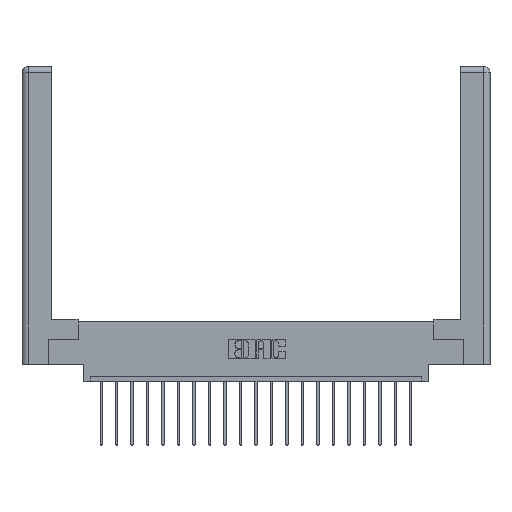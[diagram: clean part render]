
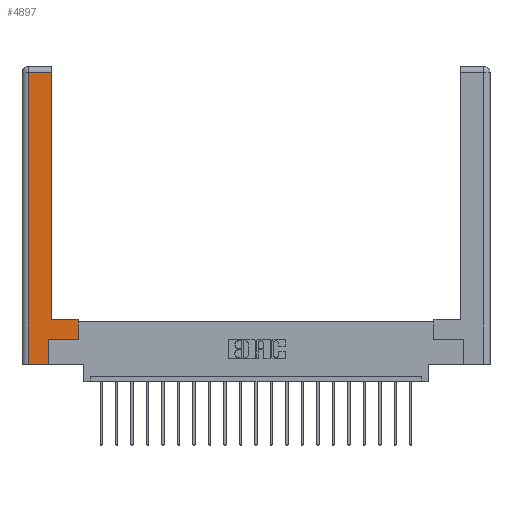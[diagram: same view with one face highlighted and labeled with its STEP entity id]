
A CAD part, top view. The second image highlights one B-rep face of the part: STEP entity #4897.
In plain terms, the highlighted planar face has unit normal (0, 0, 1).
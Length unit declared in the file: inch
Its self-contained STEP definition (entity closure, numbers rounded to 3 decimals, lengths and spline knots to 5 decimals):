
#216 = DIRECTION ( 'NONE',  ( 0., 1., 0. ) ) ;
#342 = DIRECTION ( 'NONE',  ( -1., 0., 0. ) ) ;
#1109 = LINE ( 'NONE', #13884, #18194 ) ;
#1409 = PLANE ( 'NONE',  #10050 ) ;
#1915 = EDGE_CURVE ( 'NONE', #16895, #6205, #16337, .T. ) ;
#2586 = EDGE_CURVE ( 'NONE', #8127, #14454, #13252, .T. ) ;
#2672 = CARTESIAN_POINT ( 'NONE',  ( 0.0615, 2.94, 0. ) ) ;
#2716 = LINE ( 'NONE', #16311, #3238 ) ;
#3024 = CARTESIAN_POINT ( 'NONE',  ( 0.565, 0.45, 0. ) ) ;
#3072 = CARTESIAN_POINT ( 'NONE',  ( 0., 0., 0. ) ) ;
#3238 = VECTOR ( 'NONE', #17933, 39.37008 ) ;
#4280 = LINE ( 'NONE', #17750, #5289 ) ;
#4897 = ADVANCED_FACE ( 'NONE', ( #10386 ), #1409, .F. ) ;
#4948 = LINE ( 'NONE', #17205, #15912 ) ;
#5289 = VECTOR ( 'NONE', #8028, 39.37008 ) ;
#5337 = EDGE_CURVE ( 'NONE', #16837, #8127, #4280, .T. ) ;
#6205 = VERTEX_POINT ( 'NONE', #10598 ) ;
#6308 = VERTEX_POINT ( 'NONE', #21004 ) ;
#6935 = ORIENTED_EDGE ( 'NONE', *, *, #14429, .T. ) ;
#7046 = CARTESIAN_POINT ( 'NONE',  ( 0.295, 0.45, 0. ) ) ;
#7455 = DIRECTION ( 'NONE',  ( 0., 1., 0. ) ) ;
#8028 = DIRECTION ( 'NONE',  ( 1., 0., 0. ) ) ;
#8127 = VERTEX_POINT ( 'NONE', #15616 ) ;
#8651 = CARTESIAN_POINT ( 'NONE',  ( 0.295, 3., 0. ) ) ;
#8971 = CARTESIAN_POINT ( 'NONE',  ( 0.265, 0., 0. ) ) ;
#9048 = ORIENTED_EDGE ( 'NONE', *, *, #1915, .T. ) ;
#9074 = VERTEX_POINT ( 'NONE', #13198 ) ;
#9688 = VECTOR ( 'NONE', #20368, 39.37008 ) ;
#9883 = VERTEX_POINT ( 'NONE', #7046 ) ;
#10050 = AXIS2_PLACEMENT_3D ( 'NONE', #3072, #19780, #342 ) ;
#10075 = ORIENTED_EDGE ( 'NONE', *, *, #21052, .T. ) ;
#10165 = EDGE_CURVE ( 'NONE', #6205, #16837, #4948, .T. ) ;
#10386 = FACE_OUTER_BOUND ( 'NONE', #18798, .T. ) ;
#10560 = CARTESIAN_POINT ( 'NONE',  ( 0.565, 0.45, 0. ) ) ;
#10598 = CARTESIAN_POINT ( 'NONE',  ( 0.265, 0., 0. ) ) ;
#11851 = ORIENTED_EDGE ( 'NONE', *, *, #18282, .T. ) ;
#12116 = ORIENTED_EDGE ( 'NONE', *, *, #18641, .T. ) ;
#12126 = ORIENTED_EDGE ( 'NONE', *, *, #10165, .T. ) ;
#12286 = ORIENTED_EDGE ( 'NONE', *, *, #2586, .T. ) ;
#12646 = LINE ( 'NONE', #2672, #13947 ) ;
#13198 = CARTESIAN_POINT ( 'NONE',  ( 0.295, 2.94, 0. ) ) ;
#13252 = LINE ( 'NONE', #10560, #19102 ) ;
#13451 = CARTESIAN_POINT ( 'NONE',  ( 0.0615, 0., 0. ) ) ;
#13547 = ORIENTED_EDGE ( 'NONE', *, *, #5337, .T. ) ;
#13751 = DIRECTION ( 'NONE',  ( 0., -1., 0. ) ) ;
#13884 = CARTESIAN_POINT ( 'NONE',  ( 0.0615, 0., 0. ) ) ;
#13947 = VECTOR ( 'NONE', #20822, 39.37008 ) ;
#14429 = EDGE_CURVE ( 'NONE', #9074, #6308, #12646, .T. ) ;
#14454 = VERTEX_POINT ( 'NONE', #3024 ) ;
#15616 = CARTESIAN_POINT ( 'NONE',  ( 0.565, 0.245, 0. ) ) ;
#15912 = VECTOR ( 'NONE', #19380, 39.37008 ) ;
#16311 = CARTESIAN_POINT ( 'NONE',  ( 0.295, 0.45, 0. ) ) ;
#16337 = LINE ( 'NONE', #8971, #9688 ) ;
#16837 = VERTEX_POINT ( 'NONE', #18140 ) ;
#16895 = VERTEX_POINT ( 'NONE', #13451 ) ;
#17205 = CARTESIAN_POINT ( 'NONE',  ( 0.265, 0.245, 0. ) ) ;
#17750 = CARTESIAN_POINT ( 'NONE',  ( 0.565, 0.245, 0. ) ) ;
#17933 = DIRECTION ( 'NONE',  ( -1., 0., 0. ) ) ;
#18140 = CARTESIAN_POINT ( 'NONE',  ( 0.265, 0.245, 0. ) ) ;
#18194 = VECTOR ( 'NONE', #13751, 39.37008 ) ;
#18282 = EDGE_CURVE ( 'NONE', #9883, #9074, #18744, .T. ) ;
#18641 = EDGE_CURVE ( 'NONE', #6308, #16895, #1109, .T. ) ;
#18744 = LINE ( 'NONE', #8651, #21013 ) ;
#18798 = EDGE_LOOP ( 'NONE', ( #11851, #6935, #12116, #9048, #12126, #13547, #12286, #10075 ) ) ;
#19102 = VECTOR ( 'NONE', #7455, 39.37008 ) ;
#19380 = DIRECTION ( 'NONE',  ( 0., 1., 0. ) ) ;
#19780 = DIRECTION ( 'NONE',  ( 0., 0., -1. ) ) ;
#20368 = DIRECTION ( 'NONE',  ( 1., 0., 0. ) ) ;
#20822 = DIRECTION ( 'NONE',  ( -1., 0., 0. ) ) ;
#21004 = CARTESIAN_POINT ( 'NONE',  ( 0.0615, 2.94, 0. ) ) ;
#21013 = VECTOR ( 'NONE', #216, 39.37008 ) ;
#21052 = EDGE_CURVE ( 'NONE', #14454, #9883, #2716, .T. ) ;
